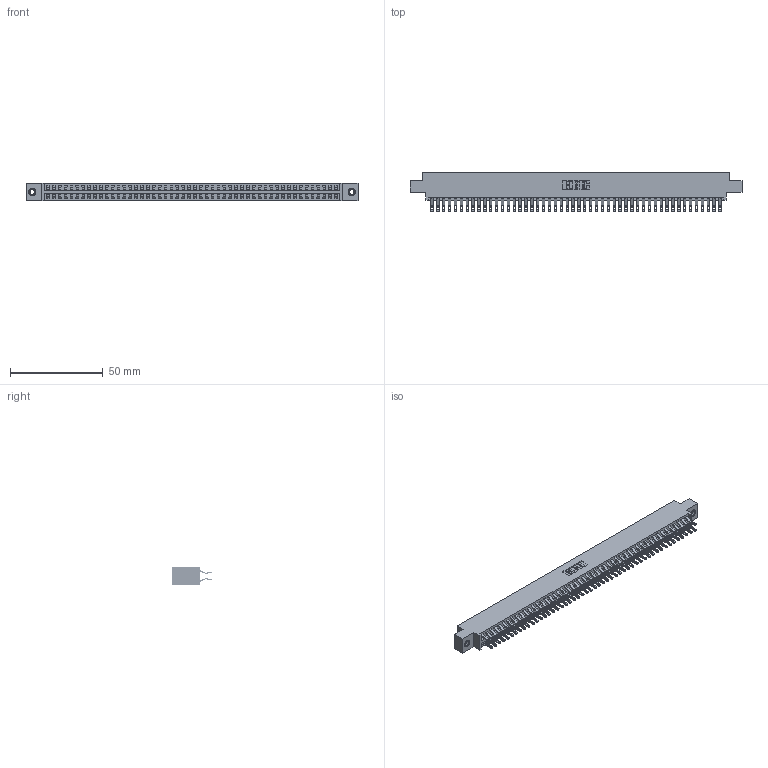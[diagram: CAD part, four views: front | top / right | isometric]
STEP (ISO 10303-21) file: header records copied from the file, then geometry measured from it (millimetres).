
FILE_DESCRIPTION (( 'STEP AP203' ), '1' );
FILE_NAME ('346-100-555-807.STEP', '2022-05-26T21:03:13', ( '' ), ( '' ), 'SwSTEP 2.0', 'SolidWorks 2020', '' );
FILE_SCHEMA (( 'CONFIG_CONTROL_DESIGN' ));
Length unit declared in the file: inch
Products named in the file (4): 346-100-555-807; 346 Part_0.170 Offset - 0.156 Dia-TI; 345-292-001_555 Tail; 345-250-001_345-250-005-103
Assembly tree (103 placements, depth 2):
  346-100-555-807
    346 Part_0.170 Offset - 0.156 Dia-TI
    345-292-001_555 Tail  x100
    345-250-001_345-250-005-103  x2
Bounding box: 179.32 x 21.46 x 9.4 mm (x, y, z)
Volume: 17670.4 mm3; surface area: 25662.2 mm2
Topology: 103 solids, 103 shells, 5986 faces, 18777 edges, 12510 vertices
Faces by surface type: plane 3412, cylinder 2558, cone 12, torus 4
Entity records: 33198 total; most frequent: CARTESIAN_POINT 5481, ORIENTED_EDGE 5378, DIRECTION 4875, EDGE_CURVE 2689, LINE 2317, VECTOR 2317, VERTEX_POINT 1788, AXIS2_PLACEMENT_3D 1279
